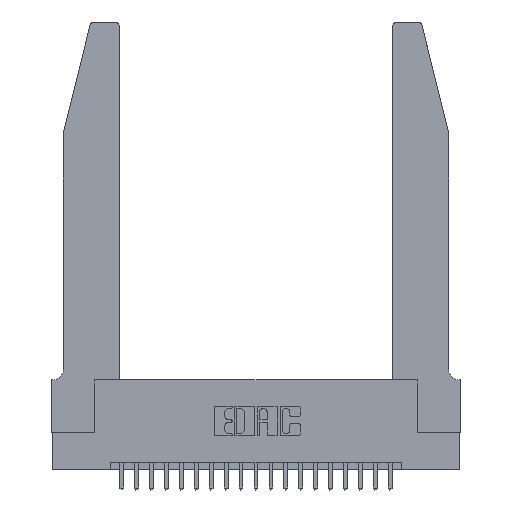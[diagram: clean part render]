
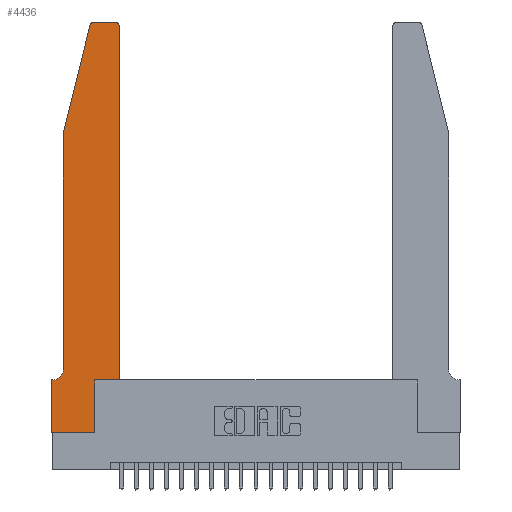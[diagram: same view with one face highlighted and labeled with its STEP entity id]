
A CAD part, top view. The second image highlights one B-rep face of the part: STEP entity #4436.
In plain terms, the highlighted planar face has unit normal (0, 0, 1).
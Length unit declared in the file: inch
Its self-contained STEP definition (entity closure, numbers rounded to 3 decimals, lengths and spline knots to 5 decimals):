
#89 = DIRECTION ( 'NONE',  ( 0., -1., 0. ) ) ;
#124 = DIRECTION ( 'NONE',  ( 1., 0., 0. ) ) ;
#756 = ORIENTED_EDGE ( 'NONE', *, *, #16251, .T. ) ;
#1241 = EDGE_CURVE ( 'NONE', #10475, #22461, #11133, .T. ) ;
#1461 = CARTESIAN_POINT ( 'NONE',  ( 0.284, 2.75, 0.37 ) ) ;
#1512 = CARTESIAN_POINT ( 'NONE',  ( 0.0755, 2., 0.37 ) ) ;
#1536 = VECTOR ( 'NONE', #14767, 39.37008 ) ;
#1763 = LINE ( 'NONE', #18476, #19944 ) ;
#2447 = AXIS2_PLACEMENT_3D ( 'NONE', #16243, #21597, #14332 ) ;
#3104 = CARTESIAN_POINT ( 'NONE',  ( 0.4505, 2.72, 0.37 ) ) ;
#3495 = LINE ( 'NONE', #19100, #4855 ) ;
#3706 = EDGE_LOOP ( 'NONE', ( #11739, #7739, #19409, #17116, #4608, #7303, #8548, #756, #3777, #22278, #4514, #11938 ) ) ;
#3759 = CARTESIAN_POINT ( 'NONE',  ( 0.4505, 0.35, 0.37 ) ) ;
#3777 = ORIENTED_EDGE ( 'NONE', *, *, #17346, .T. ) ;
#3812 = DIRECTION ( 'NONE',  ( 0., 0., 1. ) ) ;
#3818 = VERTEX_POINT ( 'NONE', #21463 ) ;
#4208 = AXIS2_PLACEMENT_3D ( 'NONE', #17914, #3812, #7503 ) ;
#4281 = DIRECTION ( 'NONE',  ( 0., -1., 0. ) ) ;
#4436 = ADVANCED_FACE ( 'NONE', ( #22576 ), #22696, .T. ) ;
#4485 = DIRECTION ( 'NONE',  ( 0., 0., 1. ) ) ;
#4514 = ORIENTED_EDGE ( 'NONE', *, *, #7390, .T. ) ;
#4579 = CARTESIAN_POINT ( 'NONE',  ( 0.0755, 0.35, 0.37 ) ) ;
#4608 = ORIENTED_EDGE ( 'NONE', *, *, #7404, .T. ) ;
#4855 = VECTOR ( 'NONE', #8785, 39.37008 ) ;
#5088 = CARTESIAN_POINT ( 'NONE',  ( 0.0055, 0.35, 0.37 ) ) ;
#5125 = VECTOR ( 'NONE', #11857, 39.37008 ) ;
#5580 = EDGE_CURVE ( 'NONE', #13675, #15524, #1763, .T. ) ;
#5893 = CARTESIAN_POINT ( 'NONE',  ( 0.4205, 2.75, 0.37 ) ) ;
#5918 = CIRCLE ( 'NONE', #15359, 0.03 ) ;
#5932 = EDGE_CURVE ( 'NONE', #22461, #3818, #11972, .T. ) ;
#6404 = CARTESIAN_POINT ( 'NONE',  ( 0.2865, 0.35, 0.37 ) ) ;
#7303 = ORIENTED_EDGE ( 'NONE', *, *, #1241, .T. ) ;
#7390 = EDGE_CURVE ( 'NONE', #14754, #16898, #20417, .T. ) ;
#7404 = EDGE_CURVE ( 'NONE', #12528, #10475, #9687, .T. ) ;
#7503 = DIRECTION ( 'NONE',  ( 1., 0., 0. ) ) ;
#7739 = ORIENTED_EDGE ( 'NONE', *, *, #22171, .T. ) ;
#8261 = CARTESIAN_POINT ( 'NONE',  ( 0.284, 2.72, 0.37 ) ) ;
#8548 = ORIENTED_EDGE ( 'NONE', *, *, #5932, .T. ) ;
#8785 = DIRECTION ( 'NONE',  ( -0.239, -0.971, 0. ) ) ;
#8879 = DIRECTION ( 'NONE',  ( 0., 0., 1. ) ) ;
#9536 = CARTESIAN_POINT ( 'NONE',  ( 0.0755, 2., 0.37 ) ) ;
#9687 = CIRCLE ( 'NONE', #2447, 0.07 ) ;
#10391 = DIRECTION ( 'NONE',  ( 0., 1., 0. ) ) ;
#10475 = VERTEX_POINT ( 'NONE', #5088 ) ;
#10508 = CARTESIAN_POINT ( 'NONE',  ( 0.25487, 2.72718, 0.37 ) ) ;
#10573 = CARTESIAN_POINT ( 'NONE',  ( 0., 0.35, 0.37 ) ) ;
#10620 = CARTESIAN_POINT ( 'NONE',  ( 0., 0., 0.37 ) ) ;
#11133 = LINE ( 'NONE', #4579, #21577 ) ;
#11194 = CARTESIAN_POINT ( 'NONE',  ( 0.0755, 0.42, 0.37 ) ) ;
#11481 = DIRECTION ( 'NONE',  ( -1., 0., 0. ) ) ;
#11739 = ORIENTED_EDGE ( 'NONE', *, *, #5580, .T. ) ;
#11857 = DIRECTION ( 'NONE',  ( 1., 0., 0. ) ) ;
#11938 = ORIENTED_EDGE ( 'NONE', *, *, #12264, .T. ) ;
#11972 = LINE ( 'NONE', #10620, #20751 ) ;
#12055 = VERTEX_POINT ( 'NONE', #10508 ) ;
#12061 = CARTESIAN_POINT ( 'NONE',  ( 0.2865, 0.35, 0.37 ) ) ;
#12264 = EDGE_CURVE ( 'NONE', #16898, #13675, #21555, .T. ) ;
#12528 = VERTEX_POINT ( 'NONE', #11194 ) ;
#12609 = LINE ( 'NONE', #22382, #5125 ) ;
#12652 = CARTESIAN_POINT ( 'NONE',  ( 0.2865, 0., 0.37 ) ) ;
#13161 = LINE ( 'NONE', #20141, #1536 ) ;
#13675 = VERTEX_POINT ( 'NONE', #5893 ) ;
#13981 = LINE ( 'NONE', #9536, #22767 ) ;
#14332 = DIRECTION ( 'NONE',  ( -1., 0., 0. ) ) ;
#14754 = VERTEX_POINT ( 'NONE', #3759 ) ;
#14767 = DIRECTION ( 'NONE',  ( 1., 0., 0. ) ) ;
#15125 = VERTEX_POINT ( 'NONE', #1512 ) ;
#15359 = AXIS2_PLACEMENT_3D ( 'NONE', #8261, #4485, #18652 ) ;
#15524 = VERTEX_POINT ( 'NONE', #1461 ) ;
#15580 = VECTOR ( 'NONE', #20648, 39.37008 ) ;
#15686 = EDGE_CURVE ( 'NONE', #12055, #15125, #3495, .T. ) ;
#15808 = VERTEX_POINT ( 'NONE', #12652 ) ;
#15891 = CARTESIAN_POINT ( 'NONE',  ( 0.4205, 2.72, 0.37 ) ) ;
#15996 = EDGE_CURVE ( 'NONE', #15125, #12528, #13981, .T. ) ;
#16017 = CARTESIAN_POINT ( 'NONE',  ( 0.4505, 0.35, 0.37 ) ) ;
#16243 = CARTESIAN_POINT ( 'NONE',  ( 0.0055, 0.42, 0.37 ) ) ;
#16251 = EDGE_CURVE ( 'NONE', #3818, #15808, #12609, .T. ) ;
#16898 = VERTEX_POINT ( 'NONE', #3104 ) ;
#16989 = VERTEX_POINT ( 'NONE', #12061 ) ;
#17116 = ORIENTED_EDGE ( 'NONE', *, *, #15996, .T. ) ;
#17346 = EDGE_CURVE ( 'NONE', #15808, #16989, #18882, .T. ) ;
#17914 = CARTESIAN_POINT ( 'NONE',  ( 0., 0.35, 0.37 ) ) ;
#18476 = CARTESIAN_POINT ( 'NONE',  ( 0.2605, 2.75, 0.37 ) ) ;
#18652 = DIRECTION ( 'NONE',  ( 1., 0., 0. ) ) ;
#18882 = LINE ( 'NONE', #6404, #15580 ) ;
#19100 = CARTESIAN_POINT ( 'NONE',  ( 0.0755, 2., 0.37 ) ) ;
#19409 = ORIENTED_EDGE ( 'NONE', *, *, #15686, .T. ) ;
#19798 = AXIS2_PLACEMENT_3D ( 'NONE', #15891, #8879, #124 ) ;
#19944 = VECTOR ( 'NONE', #11481, 39.37008 ) ;
#20141 = CARTESIAN_POINT ( 'NONE',  ( 0.4505, 0.35, 0.37 ) ) ;
#20148 = VECTOR ( 'NONE', #10391, 39.37008 ) ;
#20371 = DIRECTION ( 'NONE',  ( -1., 0., 0. ) ) ;
#20417 = LINE ( 'NONE', #16017, #20148 ) ;
#20648 = DIRECTION ( 'NONE',  ( 0., 1., 0. ) ) ;
#20751 = VECTOR ( 'NONE', #89, 39.37008 ) ;
#21463 = CARTESIAN_POINT ( 'NONE',  ( 0., 0., 0.37 ) ) ;
#21476 = EDGE_CURVE ( 'NONE', #16989, #14754, #13161, .T. ) ;
#21555 = CIRCLE ( 'NONE', #19798, 0.03 ) ;
#21577 = VECTOR ( 'NONE', #20371, 39.37008 ) ;
#21597 = DIRECTION ( 'NONE',  ( 0., 0., -1. ) ) ;
#22171 = EDGE_CURVE ( 'NONE', #15524, #12055, #5918, .T. ) ;
#22278 = ORIENTED_EDGE ( 'NONE', *, *, #21476, .T. ) ;
#22382 = CARTESIAN_POINT ( 'NONE',  ( 0., 0., 0.37 ) ) ;
#22461 = VERTEX_POINT ( 'NONE', #10573 ) ;
#22576 = FACE_OUTER_BOUND ( 'NONE', #3706, .T. ) ;
#22696 = PLANE ( 'NONE',  #4208 ) ;
#22767 = VECTOR ( 'NONE', #4281, 39.37008 ) ;
